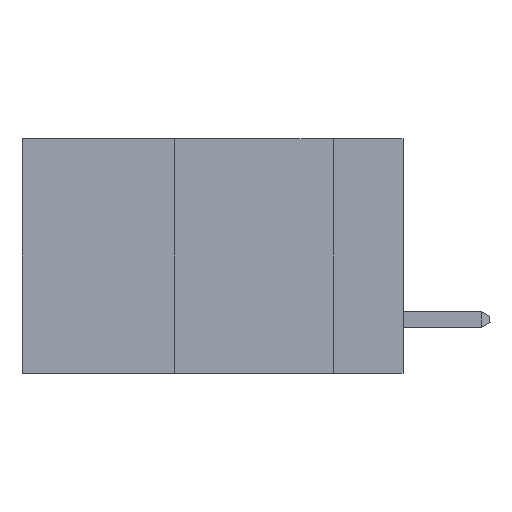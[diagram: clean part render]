
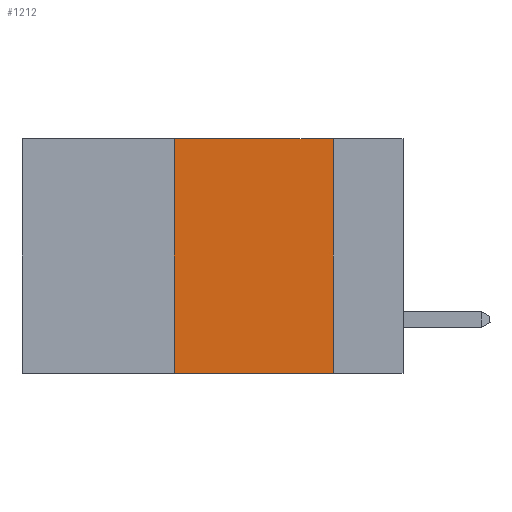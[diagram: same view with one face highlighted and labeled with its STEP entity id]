
A CAD part, left-side view. The second image highlights one B-rep face of the part: STEP entity #1212.
In plain terms, the highlighted planar face has unit normal (-1, 0, 0).
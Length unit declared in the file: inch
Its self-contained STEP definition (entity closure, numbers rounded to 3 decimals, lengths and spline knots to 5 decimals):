
#119 = CARTESIAN_POINT ( 'NONE',  ( 0., 0.36, 0. ) ) ;
#169 = ORIENTED_EDGE ( 'NONE', *, *, #3895, .F. ) ;
#261 = EDGE_CURVE ( 'NONE', #17039, #275, #13425, .T. ) ;
#275 = VERTEX_POINT ( 'NONE', #9145 ) ;
#332 = CARTESIAN_POINT ( 'NONE',  ( 0., 0.36, 0. ) ) ;
#630 = VECTOR ( 'NONE', #15315, 39.37008 ) ;
#1212 = ADVANCED_FACE ( 'NONE', ( #12047 ), #18098, .F. ) ;
#2803 = CARTESIAN_POINT ( 'NONE',  ( 0., 0.36, -0.37 ) ) ;
#3530 = CARTESIAN_POINT ( 'NONE',  ( 0., 0.11, 0. ) ) ;
#3895 = EDGE_CURVE ( 'NONE', #7440, #10035, #4606, .T. ) ;
#3991 = LINE ( 'NONE', #4695, #7150 ) ;
#4242 = VECTOR ( 'NONE', #4851, 39.37008 ) ;
#4606 = LINE ( 'NONE', #332, #630 ) ;
#4695 = CARTESIAN_POINT ( 'NONE',  ( 0., 0.6, 0. ) ) ;
#4851 = DIRECTION ( 'NONE',  ( 0., 0., -1. ) ) ;
#5389 = ORIENTED_EDGE ( 'NONE', *, *, #261, .F. ) ;
#6055 = EDGE_CURVE ( 'NONE', #10035, #17039, #3991, .T. ) ;
#6239 = DIRECTION ( 'NONE',  ( 0., -1., 0. ) ) ;
#7150 = VECTOR ( 'NONE', #6239, 39.37008 ) ;
#7440 = VERTEX_POINT ( 'NONE', #2803 ) ;
#7916 = CARTESIAN_POINT ( 'NONE',  ( 0., 0.6, -0.37 ) ) ;
#8003 = EDGE_CURVE ( 'NONE', #7440, #275, #11517, .T. ) ;
#8060 = DIRECTION ( 'NONE',  ( 1., 0., 0. ) ) ;
#8282 = CARTESIAN_POINT ( 'NONE',  ( 0., 0.6, 0. ) ) ;
#8535 = CARTESIAN_POINT ( 'NONE',  ( 0., 0.11, 0. ) ) ;
#9145 = CARTESIAN_POINT ( 'NONE',  ( 0., 0.11, -0.37 ) ) ;
#9726 = VECTOR ( 'NONE', #21581, 39.37008 ) ;
#10035 = VERTEX_POINT ( 'NONE', #119 ) ;
#11517 = LINE ( 'NONE', #7916, #9726 ) ;
#12047 = FACE_OUTER_BOUND ( 'NONE', #12925, .T. ) ;
#12925 = EDGE_LOOP ( 'NONE', ( #5389, #16110, #169, #18185 ) ) ;
#13425 = LINE ( 'NONE', #3530, #4242 ) ;
#13474 = DIRECTION ( 'NONE',  ( 0., 0., -1. ) ) ;
#15315 = DIRECTION ( 'NONE',  ( 0., 0., 1. ) ) ;
#15857 = AXIS2_PLACEMENT_3D ( 'NONE', #8282, #8060, #13474 ) ;
#16110 = ORIENTED_EDGE ( 'NONE', *, *, #6055, .F. ) ;
#17039 = VERTEX_POINT ( 'NONE', #8535 ) ;
#18098 = PLANE ( 'NONE',  #15857 ) ;
#18185 = ORIENTED_EDGE ( 'NONE', *, *, #8003, .T. ) ;
#21581 = DIRECTION ( 'NONE',  ( 0., -1., 0. ) ) ;
